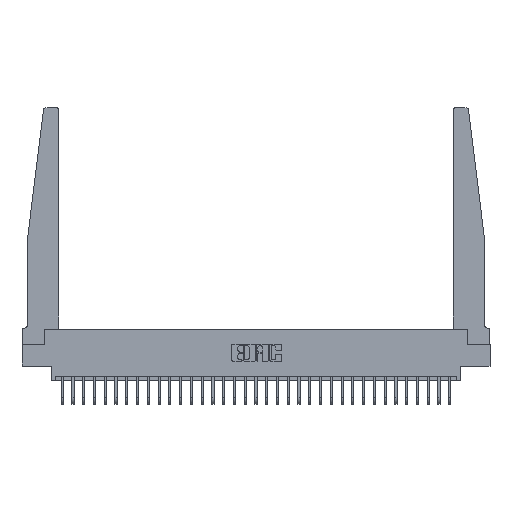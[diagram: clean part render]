
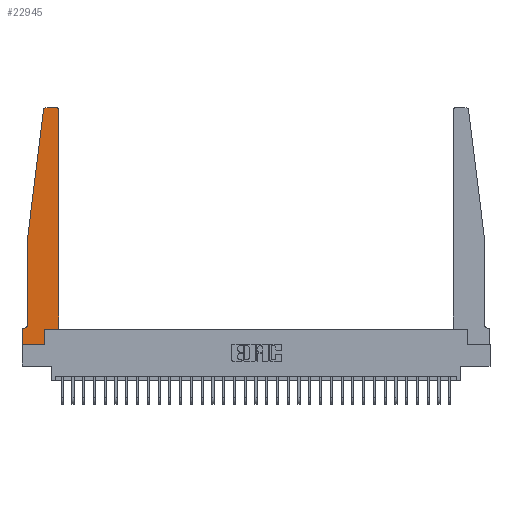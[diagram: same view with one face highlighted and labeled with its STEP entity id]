
A CAD part, top view. The second image highlights one B-rep face of the part: STEP entity #22945.
In plain terms, the highlighted planar face has unit normal (0, 0, 1).
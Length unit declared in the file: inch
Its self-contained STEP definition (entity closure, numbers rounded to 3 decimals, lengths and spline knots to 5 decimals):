
#109 = LINE ( 'NONE', #29704, #4342 ) ;
#1015 = DIRECTION ( 'NONE',  ( -1., 0., 0. ) ) ;
#1657 = DIRECTION ( 'NONE',  ( 0., 1., 0. ) ) ;
#2104 = VERTEX_POINT ( 'NONE', #10466 ) ;
#2279 = VERTEX_POINT ( 'NONE', #7707 ) ;
#2680 = DIRECTION ( 'NONE',  ( -0.122, -0.992, 0. ) ) ;
#2792 = VECTOR ( 'NONE', #2680, 39.37008 ) ;
#3329 = EDGE_LOOP ( 'NONE', ( #7407, #17359, #30256, #3353, #4191, #16131, #17756, #24754, #6224, #20092, #26299, #26604 ) ) ;
#3353 = ORIENTED_EDGE ( 'NONE', *, *, #21709, .T. ) ;
#3363 = VECTOR ( 'NONE', #1657, 39.37008 ) ;
#4191 = ORIENTED_EDGE ( 'NONE', *, *, #18237, .T. ) ;
#4342 = VECTOR ( 'NONE', #12856, 39.37008 ) ;
#4393 = EDGE_CURVE ( 'NONE', #31550, #10410, #12665, .T. ) ;
#4590 = VECTOR ( 'NONE', #22023, 39.37008 ) ;
#4767 = CARTESIAN_POINT ( 'NONE',  ( 0., 0., 0.37 ) ) ;
#4855 = LINE ( 'NONE', #12125, #4590 ) ;
#5090 = LINE ( 'NONE', #29849, #2792 ) ;
#5238 = CARTESIAN_POINT ( 'NONE',  ( 0.395, 2.72, 0.37 ) ) ;
#5866 = LINE ( 'NONE', #15769, #11711 ) ;
#5970 = DIRECTION ( 'NONE',  ( 0., 0., -1. ) ) ;
#6217 = AXIS2_PLACEMENT_3D ( 'NONE', #5238, #15151, #14826 ) ;
#6224 = ORIENTED_EDGE ( 'NONE', *, *, #10004, .T. ) ;
#6992 = VERTEX_POINT ( 'NONE', #11164 ) ;
#7407 = ORIENTED_EDGE ( 'NONE', *, *, #18402, .T. ) ;
#7707 = CARTESIAN_POINT ( 'NONE',  ( 0.395, 2.75, 0.37 ) ) ;
#9116 = VERTEX_POINT ( 'NONE', #15663 ) ;
#9379 = EDGE_CURVE ( 'NONE', #26410, #9116, #5090, .T. ) ;
#9776 = VECTOR ( 'NONE', #31395, 39.37008 ) ;
#10004 = EDGE_CURVE ( 'NONE', #10353, #16446, #21404, .T. ) ;
#10179 = VECTOR ( 'NONE', #16857, 39.37008 ) ;
#10353 = VERTEX_POINT ( 'NONE', #10958 ) ;
#10410 = VERTEX_POINT ( 'NONE', #30389 ) ;
#10466 = CARTESIAN_POINT ( 'NONE',  ( 0.065, 0.2375, 0.37 ) ) ;
#10958 = CARTESIAN_POINT ( 'NONE',  ( 0.2605, 0., 0.37 ) ) ;
#11164 = CARTESIAN_POINT ( 'NONE',  ( 0.015, 0.1875, 0.37 ) ) ;
#11394 = CARTESIAN_POINT ( 'NONE',  ( 0.24675, 2.72367, 0.37 ) ) ;
#11652 = CARTESIAN_POINT ( 'NONE',  ( 0.25, 2.75, 0.37 ) ) ;
#11711 = VECTOR ( 'NONE', #1015, 39.37008 ) ;
#11876 = VERTEX_POINT ( 'NONE', #13424 ) ;
#12080 = EDGE_CURVE ( 'NONE', #11876, #26410, #24160, .T. ) ;
#12125 = CARTESIAN_POINT ( 'NONE',  ( 0.065, 1.25, 0.37 ) ) ;
#12440 = CARTESIAN_POINT ( 'NONE',  ( 0., 0.1875, 0.37 ) ) ;
#12665 = LINE ( 'NONE', #4767, #31003 ) ;
#12856 = DIRECTION ( 'NONE',  ( 0., 1., 0. ) ) ;
#12888 = AXIS2_PLACEMENT_3D ( 'NONE', #12440, #25367, #12913 ) ;
#12913 = DIRECTION ( 'NONE',  ( 1., 0., 0. ) ) ;
#13082 = PLANE ( 'NONE',  #12888 ) ;
#13228 = VERTEX_POINT ( 'NONE', #24862 ) ;
#13424 = CARTESIAN_POINT ( 'NONE',  ( 0.27653, 2.75, 0.37 ) ) ;
#13943 = CARTESIAN_POINT ( 'NONE',  ( 0.015, 0.2375, 0.37 ) ) ;
#14581 = CARTESIAN_POINT ( 'NONE',  ( 0.27653, 2.72, 0.37 ) ) ;
#14791 = CARTESIAN_POINT ( 'NONE',  ( 0.2605, 0.18, 0.37 ) ) ;
#14826 = DIRECTION ( 'NONE',  ( 1., 0., 0. ) ) ;
#15151 = DIRECTION ( 'NONE',  ( 0., 0., 1. ) ) ;
#15214 = CARTESIAN_POINT ( 'NONE',  ( 0., 0., 0.37 ) ) ;
#15663 = CARTESIAN_POINT ( 'NONE',  ( 0.065, 1.25, 0.37 ) ) ;
#15769 = CARTESIAN_POINT ( 'NONE',  ( 0.065, 0.1875, 0.37 ) ) ;
#16131 = ORIENTED_EDGE ( 'NONE', *, *, #16378, .T. ) ;
#16378 = EDGE_CURVE ( 'NONE', #6992, #31550, #5866, .T. ) ;
#16446 = VERTEX_POINT ( 'NONE', #14791 ) ;
#16857 = DIRECTION ( 'NONE',  ( -1., 0., 0. ) ) ;
#17359 = ORIENTED_EDGE ( 'NONE', *, *, #12080, .T. ) ;
#17756 = ORIENTED_EDGE ( 'NONE', *, *, #4393, .T. ) ;
#17804 = DIRECTION ( 'NONE',  ( 1., 0., 0. ) ) ;
#18237 = EDGE_CURVE ( 'NONE', #2104, #6992, #25175, .T. ) ;
#18402 = EDGE_CURVE ( 'NONE', #2279, #11876, #29140, .T. ) ;
#20092 = ORIENTED_EDGE ( 'NONE', *, *, #22666, .T. ) ;
#20210 = FACE_OUTER_BOUND ( 'NONE', #3329, .T. ) ;
#20543 = CARTESIAN_POINT ( 'NONE',  ( 0., 0.1875, 0.37 ) ) ;
#21230 = CIRCLE ( 'NONE', #6217, 0.03 ) ;
#21404 = LINE ( 'NONE', #24143, #3363 ) ;
#21709 = EDGE_CURVE ( 'NONE', #9116, #2104, #4855, .T. ) ;
#22023 = DIRECTION ( 'NONE',  ( 0., -1., 0. ) ) ;
#22252 = DIRECTION ( 'NONE',  ( 0., -1., 0. ) ) ;
#22666 = EDGE_CURVE ( 'NONE', #16446, #22772, #26697, .T. ) ;
#22772 = VERTEX_POINT ( 'NONE', #29281 ) ;
#22945 = ADVANCED_FACE ( 'NONE', ( #20210 ), #13082, .T. ) ;
#22967 = EDGE_CURVE ( 'NONE', #10410, #10353, #29756, .T. ) ;
#23112 = AXIS2_PLACEMENT_3D ( 'NONE', #14581, #27327, #24428 ) ;
#24143 = CARTESIAN_POINT ( 'NONE',  ( 0.2605, 0.18, 0.37 ) ) ;
#24160 = CIRCLE ( 'NONE', #23112, 0.03 ) ;
#24428 = DIRECTION ( 'NONE',  ( 1., 0., 0. ) ) ;
#24446 = CARTESIAN_POINT ( 'NONE',  ( 0.425, 0.18, 0.37 ) ) ;
#24754 = ORIENTED_EDGE ( 'NONE', *, *, #22967, .T. ) ;
#24805 = VECTOR ( 'NONE', #17804, 39.37008 ) ;
#24862 = CARTESIAN_POINT ( 'NONE',  ( 0.425, 2.72, 0.37 ) ) ;
#25175 = CIRCLE ( 'NONE', #25692, 0.05 ) ;
#25204 = EDGE_CURVE ( 'NONE', #13228, #2279, #21230, .T. ) ;
#25367 = DIRECTION ( 'NONE',  ( 0., 0., 1. ) ) ;
#25692 = AXIS2_PLACEMENT_3D ( 'NONE', #13943, #5970, #28492 ) ;
#26299 = ORIENTED_EDGE ( 'NONE', *, *, #30655, .T. ) ;
#26410 = VERTEX_POINT ( 'NONE', #11394 ) ;
#26604 = ORIENTED_EDGE ( 'NONE', *, *, #25204, .T. ) ;
#26697 = LINE ( 'NONE', #24446, #9776 ) ;
#27327 = DIRECTION ( 'NONE',  ( 0., 0., 1. ) ) ;
#28492 = DIRECTION ( 'NONE',  ( -1., 0., 0. ) ) ;
#29140 = LINE ( 'NONE', #11652, #10179 ) ;
#29281 = CARTESIAN_POINT ( 'NONE',  ( 0.425, 0.18, 0.37 ) ) ;
#29704 = CARTESIAN_POINT ( 'NONE',  ( 0.425, 0.18, 0.37 ) ) ;
#29756 = LINE ( 'NONE', #15214, #24805 ) ;
#29849 = CARTESIAN_POINT ( 'NONE',  ( 0.065, 1.25, 0.37 ) ) ;
#30256 = ORIENTED_EDGE ( 'NONE', *, *, #9379, .T. ) ;
#30389 = CARTESIAN_POINT ( 'NONE',  ( 0., 0., 0.37 ) ) ;
#30655 = EDGE_CURVE ( 'NONE', #22772, #13228, #109, .T. ) ;
#31003 = VECTOR ( 'NONE', #22252, 39.37008 ) ;
#31395 = DIRECTION ( 'NONE',  ( 1., 0., 0. ) ) ;
#31550 = VERTEX_POINT ( 'NONE', #20543 ) ;
